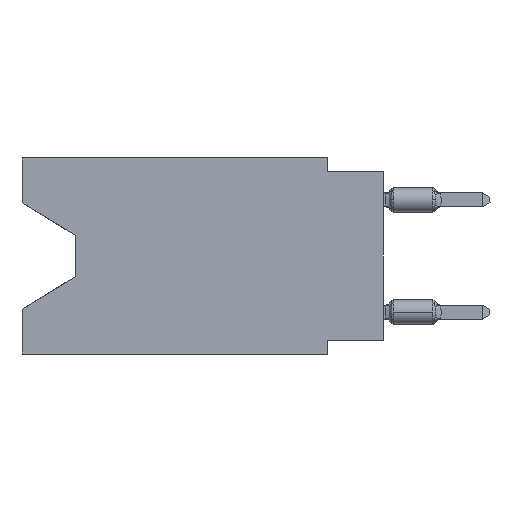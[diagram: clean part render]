
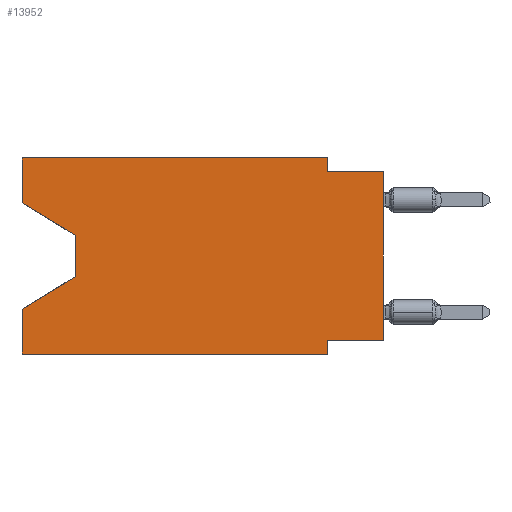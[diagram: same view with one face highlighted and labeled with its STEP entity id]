
A CAD part, left-side view. The second image highlights one B-rep face of the part: STEP entity #13952.
In plain terms, the highlighted planar face has unit normal (-1, 0, 0).
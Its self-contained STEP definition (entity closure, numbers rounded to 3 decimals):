
#161 = DIRECTION ( 'NONE',  ( 0., 0., -1. ) ) ;
#270 = CARTESIAN_POINT ( 'NONE',  ( 0., 2.54, -0.635 ) ) ;
#532 = LINE ( 'NONE', #2030, #12941 ) ;
#751 = CARTESIAN_POINT ( 'NONE',  ( 0., 0., -0.635 ) ) ;
#800 = EDGE_CURVE ( 'NONE', #3935, #8564, #3075, .T. ) ;
#1211 = VERTEX_POINT ( 'NONE', #6391 ) ;
#1444 = DIRECTION ( 'NONE',  ( 0., 0., 1. ) ) ;
#1702 = ORIENTED_EDGE ( 'NONE', *, *, #800, .F. ) ;
#1846 = VECTOR ( 'NONE', #1444, 1000. ) ;
#1928 = VERTEX_POINT ( 'NONE', #270 ) ;
#1984 = CARTESIAN_POINT ( 'NONE',  ( 0., 16.383, -6.852 ) ) ;
#2030 = CARTESIAN_POINT ( 'NONE',  ( 0., 0., -8.255 ) ) ;
#2105 = VERTEX_POINT ( 'NONE', #1984 ) ;
#2195 = VECTOR ( 'NONE', #8854, 1000. ) ;
#2244 = CARTESIAN_POINT ( 'NONE',  ( 0., 0., 0. ) ) ;
#2366 = CARTESIAN_POINT ( 'NONE',  ( 0., 16.383, 0. ) ) ;
#2528 = FACE_OUTER_BOUND ( 'NONE', #13335, .T. ) ;
#2636 = EDGE_CURVE ( 'NONE', #9927, #2105, #6599, .T. ) ;
#2651 = EDGE_CURVE ( 'NONE', #1211, #9927, #7719, .T. ) ;
#2995 = CARTESIAN_POINT ( 'NONE',  ( 0., 2.54, -8.89 ) ) ;
#3075 = LINE ( 'NONE', #12616, #10380 ) ;
#3134 = LINE ( 'NONE', #3202, #3508 ) ;
#3202 = CARTESIAN_POINT ( 'NONE',  ( 0., 16.383, -8.89 ) ) ;
#3493 = VERTEX_POINT ( 'NONE', #7620 ) ;
#3508 = VECTOR ( 'NONE', #12885, 1000. ) ;
#3535 = ORIENTED_EDGE ( 'NONE', *, *, #5683, .F. ) ;
#3562 = VERTEX_POINT ( 'NONE', #6906 ) ;
#3842 = VERTEX_POINT ( 'NONE', #8455 ) ;
#3935 = VERTEX_POINT ( 'NONE', #6478 ) ;
#3938 = DIRECTION ( 'NONE',  ( 0., -0.855, -0.519 ) ) ;
#3982 = VECTOR ( 'NONE', #12957, 1000. ) ;
#3989 = DIRECTION ( 'NONE',  ( 0., 0., 1. ) ) ;
#4075 = VECTOR ( 'NONE', #8644, 1000. ) ;
#4077 = ORIENTED_EDGE ( 'NONE', *, *, #2651, .T. ) ;
#4334 = LINE ( 'NONE', #2995, #5558 ) ;
#4474 = AXIS2_PLACEMENT_3D ( 'NONE', #9806, #6834, #7615 ) ;
#4618 = ORIENTED_EDGE ( 'NONE', *, *, #12608, .T. ) ;
#4750 = ORIENTED_EDGE ( 'NONE', *, *, #9388, .F. ) ;
#4863 = DIRECTION ( 'NONE',  ( 0., 1., 0. ) ) ;
#5405 = CARTESIAN_POINT ( 'NONE',  ( 0., 0., -0.635 ) ) ;
#5479 = LINE ( 'NONE', #2366, #11784 ) ;
#5558 = VECTOR ( 'NONE', #8635, 1000. ) ;
#5592 = VECTOR ( 'NONE', #3938, 1000. ) ;
#5683 = EDGE_CURVE ( 'NONE', #1928, #11671, #8579, .T. ) ;
#5867 = CARTESIAN_POINT ( 'NONE',  ( 0., 16.383, 0. ) ) ;
#6001 = LINE ( 'NONE', #6069, #5592 ) ;
#6069 = CARTESIAN_POINT ( 'NONE',  ( 0., 16.383, -2.038 ) ) ;
#6255 = ORIENTED_EDGE ( 'NONE', *, *, #10915, .F. ) ;
#6317 = ORIENTED_EDGE ( 'NONE', *, *, #7798, .F. ) ;
#6383 = VECTOR ( 'NONE', #161, 1000. ) ;
#6391 = CARTESIAN_POINT ( 'NONE',  ( 0., 13.97, -3.505 ) ) ;
#6478 = CARTESIAN_POINT ( 'NONE',  ( 0., 16.383, -2.038 ) ) ;
#6599 = LINE ( 'NONE', #10905, #2195 ) ;
#6788 = EDGE_CURVE ( 'NONE', #8564, #3493, #5479, .T. ) ;
#6834 = DIRECTION ( 'NONE',  ( 1., 0., 0. ) ) ;
#6906 = CARTESIAN_POINT ( 'NONE',  ( 0., 2.54, -8.255 ) ) ;
#6912 = DIRECTION ( 'NONE',  ( 0., 0., 1. ) ) ;
#7122 = CARTESIAN_POINT ( 'NONE',  ( 0., 13.97, -5.385 ) ) ;
#7391 = CARTESIAN_POINT ( 'NONE',  ( 0., 16.383, -8.89 ) ) ;
#7615 = DIRECTION ( 'NONE',  ( 0., 0., -1. ) ) ;
#7620 = CARTESIAN_POINT ( 'NONE',  ( 0., 2.54, 0. ) ) ;
#7664 = EDGE_CURVE ( 'NONE', #9259, #2105, #9039, .T. ) ;
#7665 = LINE ( 'NONE', #11900, #6383 ) ;
#7719 = LINE ( 'NONE', #8643, #3982 ) ;
#7798 = EDGE_CURVE ( 'NONE', #8501, #3562, #532, .T. ) ;
#8045 = ORIENTED_EDGE ( 'NONE', *, *, #6788, .F. ) ;
#8264 = ORIENTED_EDGE ( 'NONE', *, *, #7664, .F. ) ;
#8455 = CARTESIAN_POINT ( 'NONE',  ( 0., 2.54, -8.89 ) ) ;
#8501 = VERTEX_POINT ( 'NONE', #10049 ) ;
#8564 = VERTEX_POINT ( 'NONE', #10117 ) ;
#8579 = LINE ( 'NONE', #5405, #4075 ) ;
#8635 = DIRECTION ( 'NONE',  ( 0., 0., -1. ) ) ;
#8643 = CARTESIAN_POINT ( 'NONE',  ( 0., 13.97, -3.505 ) ) ;
#8644 = DIRECTION ( 'NONE',  ( 0., -1., 0. ) ) ;
#8713 = ORIENTED_EDGE ( 'NONE', *, *, #2636, .T. ) ;
#8715 = DIRECTION ( 'NONE',  ( 0., -1., 0. ) ) ;
#8729 = ORIENTED_EDGE ( 'NONE', *, *, #9405, .T. ) ;
#8854 = DIRECTION ( 'NONE',  ( 0., 0.855, -0.519 ) ) ;
#8877 = VECTOR ( 'NONE', #6912, 1000. ) ;
#9039 = LINE ( 'NONE', #5867, #8877 ) ;
#9259 = VERTEX_POINT ( 'NONE', #7391 ) ;
#9388 = EDGE_CURVE ( 'NONE', #3493, #1928, #7665, .T. ) ;
#9405 = EDGE_CURVE ( 'NONE', #8501, #11671, #10850, .T. ) ;
#9806 = CARTESIAN_POINT ( 'NONE',  ( 0., 16.383, 0. ) ) ;
#9927 = VERTEX_POINT ( 'NONE', #7122 ) ;
#10049 = CARTESIAN_POINT ( 'NONE',  ( 0., 0., -8.255 ) ) ;
#10117 = CARTESIAN_POINT ( 'NONE',  ( 0., 16.383, 0. ) ) ;
#10343 = ORIENTED_EDGE ( 'NONE', *, *, #10838, .T. ) ;
#10380 = VECTOR ( 'NONE', #3989, 1000. ) ;
#10838 = EDGE_CURVE ( 'NONE', #9259, #3842, #3134, .T. ) ;
#10850 = LINE ( 'NONE', #2244, #1846 ) ;
#10905 = CARTESIAN_POINT ( 'NONE',  ( 0., 13.97, -5.385 ) ) ;
#10915 = EDGE_CURVE ( 'NONE', #3562, #3842, #4334, .T. ) ;
#11671 = VERTEX_POINT ( 'NONE', #751 ) ;
#11784 = VECTOR ( 'NONE', #8715, 1000. ) ;
#11900 = CARTESIAN_POINT ( 'NONE',  ( 0., 2.54, 0. ) ) ;
#12608 = EDGE_CURVE ( 'NONE', #3935, #1211, #6001, .T. ) ;
#12616 = CARTESIAN_POINT ( 'NONE',  ( 0., 16.383, 0. ) ) ;
#12885 = DIRECTION ( 'NONE',  ( 0., -1., 0. ) ) ;
#12941 = VECTOR ( 'NONE', #4863, 1000. ) ;
#12957 = DIRECTION ( 'NONE',  ( 0., 0., -1. ) ) ;
#13056 = PLANE ( 'NONE',  #4474 ) ;
#13335 = EDGE_LOOP ( 'NONE', ( #4618, #4077, #8713, #8264, #10343, #6255, #6317, #8729, #3535, #4750, #8045, #1702 ) ) ;
#13952 = ADVANCED_FACE ( 'NONE', ( #2528 ), #13056, .F. ) ;
